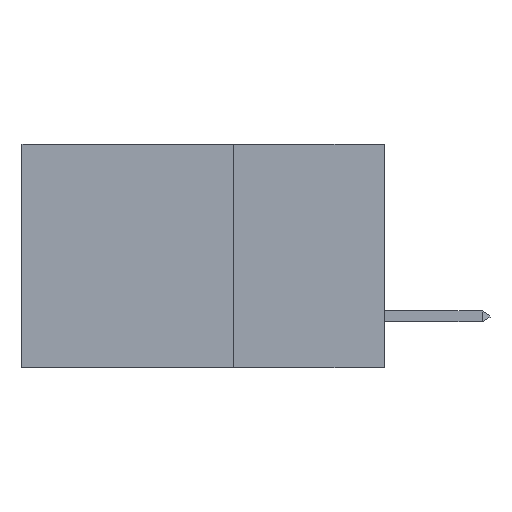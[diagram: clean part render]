
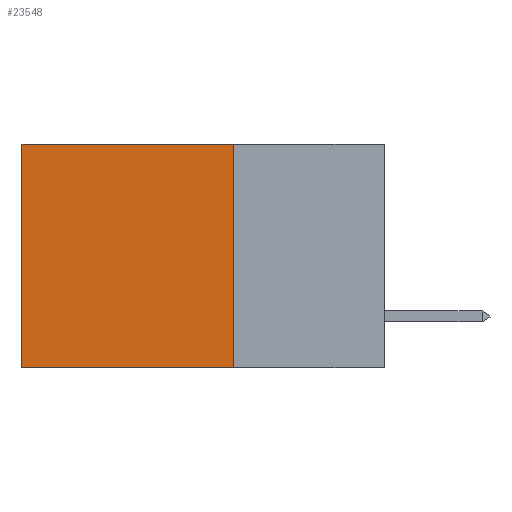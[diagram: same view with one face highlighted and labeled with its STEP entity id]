
A CAD part, left-side view. The second image highlights one B-rep face of the part: STEP entity #23548.
In plain terms, the highlighted planar face has unit normal (-1, 0, 0).
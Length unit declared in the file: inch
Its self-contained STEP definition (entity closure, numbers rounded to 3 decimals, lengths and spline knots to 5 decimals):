
#779 = EDGE_LOOP ( 'NONE', ( #19689, #30438, #8552, #2273 ) ) ;
#2273 = ORIENTED_EDGE ( 'NONE', *, *, #27139, .T. ) ;
#3964 = EDGE_CURVE ( 'NONE', #12566, #18637, #20204, .T. ) ;
#5710 = VECTOR ( 'NONE', #8306, 39.37008 ) ;
#6181 = CARTESIAN_POINT ( 'NONE',  ( 0.2875, 0.6, 0. ) ) ;
#7295 = VERTEX_POINT ( 'NONE', #17228 ) ;
#7451 = VERTEX_POINT ( 'NONE', #13019 ) ;
#8306 = DIRECTION ( 'NONE',  ( 0., 1., 0. ) ) ;
#8552 = ORIENTED_EDGE ( 'NONE', *, *, #17541, .F. ) ;
#10977 = DIRECTION ( 'NONE',  ( 0., 0., -1. ) ) ;
#12566 = VERTEX_POINT ( 'NONE', #26372 ) ;
#13019 = CARTESIAN_POINT ( 'NONE',  ( 0.2875, 0.25, 0. ) ) ;
#13278 = DIRECTION ( 'NONE',  ( 0., 0., -1. ) ) ;
#15573 = CARTESIAN_POINT ( 'NONE',  ( 0.2875, 0.25, -0.37 ) ) ;
#15577 = CARTESIAN_POINT ( 'NONE',  ( 0.2875, 0.25, 0. ) ) ;
#16489 = EDGE_CURVE ( 'NONE', #7295, #18637, #24406, .T. ) ;
#16608 = LINE ( 'NONE', #31604, #28144 ) ;
#17228 = CARTESIAN_POINT ( 'NONE',  ( 0.2875, 0.25, -0.37 ) ) ;
#17541 = EDGE_CURVE ( 'NONE', #7451, #7295, #18119, .T. ) ;
#18119 = LINE ( 'NONE', #25572, #31240 ) ;
#18637 = VERTEX_POINT ( 'NONE', #24977 ) ;
#19689 = ORIENTED_EDGE ( 'NONE', *, *, #3964, .T. ) ;
#20204 = LINE ( 'NONE', #6181, #26001 ) ;
#20710 = FACE_OUTER_BOUND ( 'NONE', #779, .T. ) ;
#21931 = AXIS2_PLACEMENT_3D ( 'NONE', #15577, #27936, #13278 ) ;
#23022 = PLANE ( 'NONE',  #21931 ) ;
#23213 = DIRECTION ( 'NONE',  ( 0., 0., -1. ) ) ;
#23548 = ADVANCED_FACE ( 'NONE', ( #20710 ), #23022, .F. ) ;
#24406 = LINE ( 'NONE', #15573, #5710 ) ;
#24977 = CARTESIAN_POINT ( 'NONE',  ( 0.2875, 0.6, -0.37 ) ) ;
#25572 = CARTESIAN_POINT ( 'NONE',  ( 0.2875, 0.25, 0. ) ) ;
#26001 = VECTOR ( 'NONE', #23213, 39.37008 ) ;
#26372 = CARTESIAN_POINT ( 'NONE',  ( 0.2875, 0.6, 0. ) ) ;
#27139 = EDGE_CURVE ( 'NONE', #7451, #12566, #16608, .T. ) ;
#27936 = DIRECTION ( 'NONE',  ( 1., 0., 0. ) ) ;
#28144 = VECTOR ( 'NONE', #29328, 39.37008 ) ;
#29328 = DIRECTION ( 'NONE',  ( 0., 1., 0. ) ) ;
#30438 = ORIENTED_EDGE ( 'NONE', *, *, #16489, .F. ) ;
#31240 = VECTOR ( 'NONE', #10977, 39.37008 ) ;
#31604 = CARTESIAN_POINT ( 'NONE',  ( 0.2875, 0.25, 0. ) ) ;
